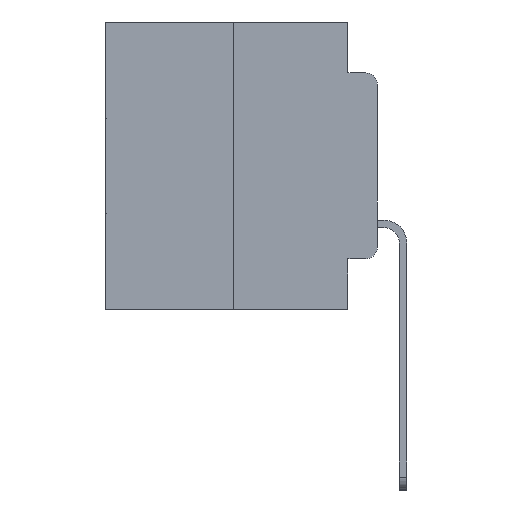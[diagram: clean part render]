
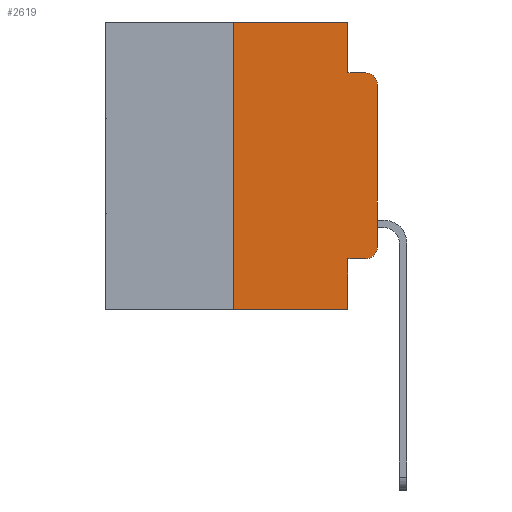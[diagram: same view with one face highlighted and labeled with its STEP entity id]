
A CAD part, left-side view. The second image highlights one B-rep face of the part: STEP entity #2619.
In plain terms, the highlighted planar face has unit normal (-1, 0, 0).
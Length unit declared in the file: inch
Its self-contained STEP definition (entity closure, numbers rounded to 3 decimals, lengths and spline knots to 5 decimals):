
#1222 = CARTESIAN_POINT ( 'NONE',  ( 0., 0.051, -0.0885 ) ) ;
#1361 = CARTESIAN_POINT ( 'NONE',  ( 0., 0., -0.3915 ) ) ;
#1698 = EDGE_LOOP ( 'NONE', ( #14775, #5265, #16580, #4913, #4663, #27735, #7386, #3898, #10996, #8882 ) ) ;
#2155 = CARTESIAN_POINT ( 'NONE',  ( 0., 0., 0. ) ) ;
#2158 = CIRCLE ( 'NONE', #3720, 0.02 ) ;
#2429 = CARTESIAN_POINT ( 'NONE',  ( 0., 0.02, -0.0885 ) ) ;
#2619 = ADVANCED_FACE ( 'NONE', ( #5987 ), #28015, .F. ) ;
#2631 = CARTESIAN_POINT ( 'NONE',  ( 0., 0.02, -0.1085 ) ) ;
#2705 = CARTESIAN_POINT ( 'NONE',  ( 0., 0.051, 0. ) ) ;
#3312 = LINE ( 'NONE', #6108, #26038 ) ;
#3683 = VERTEX_POINT ( 'NONE', #1361 ) ;
#3720 = AXIS2_PLACEMENT_3D ( 'NONE', #18160, #4823, #20333 ) ;
#3898 = ORIENTED_EDGE ( 'NONE', *, *, #22398, .F. ) ;
#4056 = EDGE_CURVE ( 'NONE', #6072, #24042, #23437, .T. ) ;
#4663 = ORIENTED_EDGE ( 'NONE', *, *, #18207, .F. ) ;
#4823 = DIRECTION ( 'NONE',  ( -1., 0., 0. ) ) ;
#4913 = ORIENTED_EDGE ( 'NONE', *, *, #15274, .F. ) ;
#4952 = DIRECTION ( 'NONE',  ( 0., 0., -1. ) ) ;
#5066 = LINE ( 'NONE', #5363, #10387 ) ;
#5265 = ORIENTED_EDGE ( 'NONE', *, *, #22184, .T. ) ;
#5363 = CARTESIAN_POINT ( 'NONE',  ( 0., 0.25, 0. ) ) ;
#5681 = VERTEX_POINT ( 'NONE', #1222 ) ;
#5987 = FACE_OUTER_BOUND ( 'NONE', #1698, .T. ) ;
#6072 = VERTEX_POINT ( 'NONE', #18388 ) ;
#6108 = CARTESIAN_POINT ( 'NONE',  ( 0., 0.473, 0. ) ) ;
#6148 = LINE ( 'NONE', #12618, #17281 ) ;
#6490 = CARTESIAN_POINT ( 'NONE',  ( 0., 0.02, -0.4115 ) ) ;
#6670 = CARTESIAN_POINT ( 'NONE',  ( 0., 0.25, 0. ) ) ;
#7167 = LINE ( 'NONE', #21445, #11038 ) ;
#7337 = VECTOR ( 'NONE', #27535, 39.37008 ) ;
#7386 = ORIENTED_EDGE ( 'NONE', *, *, #24508, .T. ) ;
#8047 = VERTEX_POINT ( 'NONE', #2429 ) ;
#8382 = AXIS2_PLACEMENT_3D ( 'NONE', #22888, #23373, #27873 ) ;
#8482 = DIRECTION ( 'NONE',  ( 0., -1., 0. ) ) ;
#8882 = ORIENTED_EDGE ( 'NONE', *, *, #16968, .T. ) ;
#10387 = VECTOR ( 'NONE', #16482, 39.37008 ) ;
#10996 = ORIENTED_EDGE ( 'NONE', *, *, #4056, .T. ) ;
#11038 = VECTOR ( 'NONE', #19283, 39.37008 ) ;
#11854 = VERTEX_POINT ( 'NONE', #6670 ) ;
#12618 = CARTESIAN_POINT ( 'NONE',  ( 0., 0.473, -0.5 ) ) ;
#13569 = LINE ( 'NONE', #2705, #18707 ) ;
#13969 = LINE ( 'NONE', #18940, #7337 ) ;
#14775 = ORIENTED_EDGE ( 'NONE', *, *, #24131, .T. ) ;
#15067 = VERTEX_POINT ( 'NONE', #25514 ) ;
#15274 = EDGE_CURVE ( 'NONE', #21739, #5681, #13569, .T. ) ;
#16482 = DIRECTION ( 'NONE',  ( 0., 0., 1. ) ) ;
#16580 = ORIENTED_EDGE ( 'NONE', *, *, #17309, .F. ) ;
#16718 = DIRECTION ( 'NONE',  ( 0., -1., 0. ) ) ;
#16968 = EDGE_CURVE ( 'NONE', #24042, #3683, #2158, .T. ) ;
#17281 = VECTOR ( 'NONE', #25576, 39.37008 ) ;
#17309 = EDGE_CURVE ( 'NONE', #5681, #8047, #7167, .T. ) ;
#18160 = CARTESIAN_POINT ( 'NONE',  ( 0., 0.02, -0.3915 ) ) ;
#18207 = EDGE_CURVE ( 'NONE', #11854, #21739, #3312, .T. ) ;
#18284 = DIRECTION ( 'NONE',  ( -1., 0., 0. ) ) ;
#18388 = CARTESIAN_POINT ( 'NONE',  ( 0., 0.051, -0.4115 ) ) ;
#18707 = VECTOR ( 'NONE', #20528, 39.37008 ) ;
#18759 = CIRCLE ( 'NONE', #27702, 0.02 ) ;
#18940 = CARTESIAN_POINT ( 'NONE',  ( 0., 0.051, 0. ) ) ;
#19283 = DIRECTION ( 'NONE',  ( 0., -1., 0. ) ) ;
#19988 = DIRECTION ( 'NONE',  ( 0., 0., 1. ) ) ;
#20333 = DIRECTION ( 'NONE',  ( 0., 0., -1. ) ) ;
#20528 = DIRECTION ( 'NONE',  ( 0., 0., -1. ) ) ;
#20727 = CARTESIAN_POINT ( 'NONE',  ( 0., 0.051, -0.5 ) ) ;
#20958 = CARTESIAN_POINT ( 'NONE',  ( 0., 0.051, 0. ) ) ;
#21058 = CARTESIAN_POINT ( 'NONE',  ( 0., 0., -0.1085 ) ) ;
#21445 = CARTESIAN_POINT ( 'NONE',  ( 0., 0.051, -0.0885 ) ) ;
#21739 = VERTEX_POINT ( 'NONE', #20958 ) ;
#22184 = EDGE_CURVE ( 'NONE', #25575, #8047, #18759, .T. ) ;
#22398 = EDGE_CURVE ( 'NONE', #6072, #28034, #13969, .T. ) ;
#22786 = VECTOR ( 'NONE', #16718, 39.37008 ) ;
#22888 = CARTESIAN_POINT ( 'NONE',  ( 0., 0.473, 0. ) ) ;
#23033 = VECTOR ( 'NONE', #19988, 39.37008 ) ;
#23226 = CARTESIAN_POINT ( 'NONE',  ( 0., 0.051, -0.4115 ) ) ;
#23373 = DIRECTION ( 'NONE',  ( 1., 0., 0. ) ) ;
#23437 = LINE ( 'NONE', #23226, #22786 ) ;
#24042 = VERTEX_POINT ( 'NONE', #6490 ) ;
#24131 = EDGE_CURVE ( 'NONE', #3683, #25575, #28012, .T. ) ;
#24348 = EDGE_CURVE ( 'NONE', #15067, #11854, #5066, .T. ) ;
#24508 = EDGE_CURVE ( 'NONE', #15067, #28034, #6148, .T. ) ;
#25514 = CARTESIAN_POINT ( 'NONE',  ( 0., 0.25, -0.5 ) ) ;
#25575 = VERTEX_POINT ( 'NONE', #21058 ) ;
#25576 = DIRECTION ( 'NONE',  ( 0., -1., 0. ) ) ;
#26038 = VECTOR ( 'NONE', #8482, 39.37008 ) ;
#27535 = DIRECTION ( 'NONE',  ( 0., 0., -1. ) ) ;
#27702 = AXIS2_PLACEMENT_3D ( 'NONE', #2631, #18284, #4952 ) ;
#27735 = ORIENTED_EDGE ( 'NONE', *, *, #24348, .F. ) ;
#27873 = DIRECTION ( 'NONE',  ( 0., 0., -1. ) ) ;
#28012 = LINE ( 'NONE', #2155, #23033 ) ;
#28015 = PLANE ( 'NONE',  #8382 ) ;
#28034 = VERTEX_POINT ( 'NONE', #20727 ) ;
